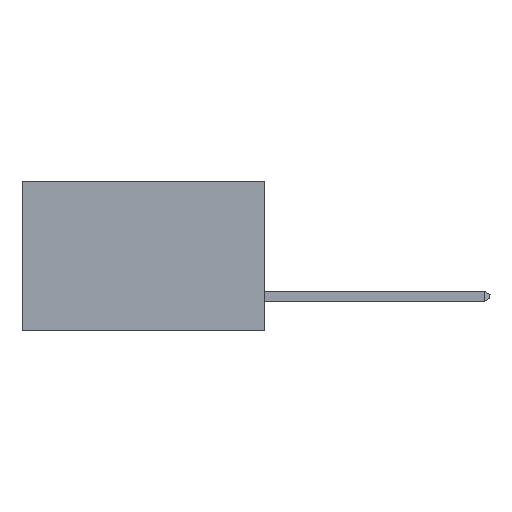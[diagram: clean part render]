
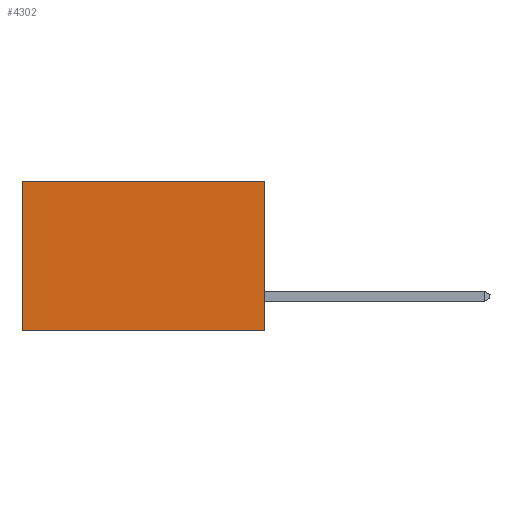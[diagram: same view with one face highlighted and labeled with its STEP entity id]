
A CAD part, left-side view. The second image highlights one B-rep face of the part: STEP entity #4302.
In plain terms, the highlighted planar face has unit normal (-1, 0, 0).
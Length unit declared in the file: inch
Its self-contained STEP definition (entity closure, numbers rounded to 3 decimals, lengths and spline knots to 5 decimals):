
#2762 = CARTESIAN_POINT ( 'NONE',  ( 0.298, 0.6, 0. ) ) ;
#3316 = DIRECTION ( 'NONE',  ( 0., 0., -1. ) ) ;
#3434 = LINE ( 'NONE', #13920, #14588 ) ;
#3435 = FACE_OUTER_BOUND ( 'NONE', #5417, .T. ) ;
#3438 = ORIENTED_EDGE ( 'NONE', *, *, #12833, .T. ) ;
#3671 = ORIENTED_EDGE ( 'NONE', *, *, #16384, .T. ) ;
#4302 = ADVANCED_FACE ( 'NONE', ( #3435 ), #8864, .F. ) ;
#5159 = DIRECTION ( 'NONE',  ( 1., 0., 0. ) ) ;
#5417 = EDGE_LOOP ( 'NONE', ( #3438, #16204, #11367, #3671 ) ) ;
#5590 = VERTEX_POINT ( 'NONE', #2762 ) ;
#6196 = CARTESIAN_POINT ( 'NONE',  ( 0.298, 0.6, -0.37 ) ) ;
#6209 = VERTEX_POINT ( 'NONE', #6196 ) ;
#6669 = AXIS2_PLACEMENT_3D ( 'NONE', #9925, #5159, #15021 ) ;
#7482 = VECTOR ( 'NONE', #8693, 39.37008 ) ;
#8386 = VERTEX_POINT ( 'NONE', #9210 ) ;
#8519 = CARTESIAN_POINT ( 'NONE',  ( 0.298, 0., 0. ) ) ;
#8632 = DIRECTION ( 'NONE',  ( 0., 0., -1. ) ) ;
#8693 = DIRECTION ( 'NONE',  ( 0., 1., 0. ) ) ;
#8864 = PLANE ( 'NONE',  #6669 ) ;
#8994 = DIRECTION ( 'NONE',  ( 0., 1., 0. ) ) ;
#9210 = CARTESIAN_POINT ( 'NONE',  ( 0.298, 0., -0.37 ) ) ;
#9776 = VECTOR ( 'NONE', #8632, 39.37008 ) ;
#9925 = CARTESIAN_POINT ( 'NONE',  ( 0.298, 0., 0. ) ) ;
#10628 = EDGE_CURVE ( 'NONE', #8386, #6209, #13206, .T. ) ;
#10803 = LINE ( 'NONE', #8519, #9776 ) ;
#11315 = EDGE_CURVE ( 'NONE', #11511, #8386, #10803, .T. ) ;
#11367 = ORIENTED_EDGE ( 'NONE', *, *, #11315, .F. ) ;
#11511 = VERTEX_POINT ( 'NONE', #16843 ) ;
#12833 = EDGE_CURVE ( 'NONE', #5590, #6209, #3434, .T. ) ;
#13015 = CARTESIAN_POINT ( 'NONE',  ( 0.298, 0., -0.37 ) ) ;
#13206 = LINE ( 'NONE', #13015, #7482 ) ;
#13820 = VECTOR ( 'NONE', #8994, 39.37008 ) ;
#13920 = CARTESIAN_POINT ( 'NONE',  ( 0.298, 0.6, 0. ) ) ;
#14031 = LINE ( 'NONE', #15802, #13820 ) ;
#14588 = VECTOR ( 'NONE', #3316, 39.37008 ) ;
#15021 = DIRECTION ( 'NONE',  ( 0., 0., -1. ) ) ;
#15802 = CARTESIAN_POINT ( 'NONE',  ( 0.298, 0., 0. ) ) ;
#16204 = ORIENTED_EDGE ( 'NONE', *, *, #10628, .F. ) ;
#16384 = EDGE_CURVE ( 'NONE', #11511, #5590, #14031, .T. ) ;
#16843 = CARTESIAN_POINT ( 'NONE',  ( 0.298, 0., 0. ) ) ;
